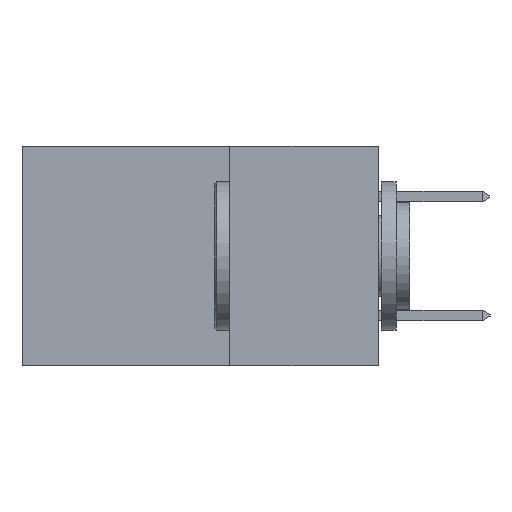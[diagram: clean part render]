
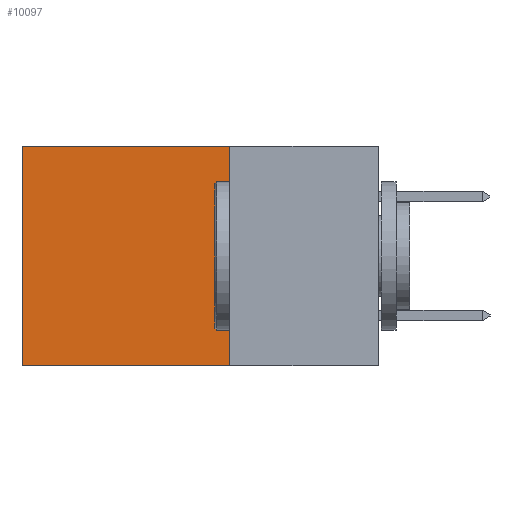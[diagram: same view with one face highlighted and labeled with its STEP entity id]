
A CAD part, left-side view. The second image highlights one B-rep face of the part: STEP entity #10097.
In plain terms, the highlighted planar face has unit normal (-1, 0, 0).
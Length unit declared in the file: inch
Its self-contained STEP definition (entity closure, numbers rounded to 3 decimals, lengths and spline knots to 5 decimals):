
#1505 = FACE_OUTER_BOUND ( 'NONE', #16225, .T. ) ;
#1739 = ORIENTED_EDGE ( 'NONE', *, *, #15482, .F. ) ;
#2769 = LINE ( 'NONE', #20878, #15574 ) ;
#2841 = EDGE_CURVE ( 'NONE', #17433, #18248, #5862, .T. ) ;
#3151 = LINE ( 'NONE', #16389, #19868 ) ;
#4175 = DIRECTION ( 'NONE',  ( 0., 1., 0. ) ) ;
#5307 = PLANE ( 'NONE',  #9100 ) ;
#5490 = VERTEX_POINT ( 'NONE', #20787 ) ;
#5681 = ORIENTED_EDGE ( 'NONE', *, *, #12714, .T. ) ;
#5862 = LINE ( 'NONE', #15817, #18675 ) ;
#6320 = CARTESIAN_POINT ( 'NONE',  ( 0.2615, 0.6, -0.37 ) ) ;
#7467 = CARTESIAN_POINT ( 'NONE',  ( 0.2615, 0.6, 0. ) ) ;
#8019 = DIRECTION ( 'NONE',  ( 0., 0., -1. ) ) ;
#8692 = DIRECTION ( 'NONE',  ( 0., 0., -1. ) ) ;
#8727 = LINE ( 'NONE', #6320, #17052 ) ;
#9100 = AXIS2_PLACEMENT_3D ( 'NONE', #16976, #18687, #8692 ) ;
#10097 = ADVANCED_FACE ( 'NONE', ( #1505 ), #5307, .F. ) ;
#11141 = EDGE_CURVE ( 'NONE', #5490, #21105, #2769, .T. ) ;
#12714 = EDGE_CURVE ( 'NONE', #18248, #21105, #8727, .T. ) ;
#13127 = DIRECTION ( 'NONE',  ( 0., 0., -1. ) ) ;
#15156 = ORIENTED_EDGE ( 'NONE', *, *, #2841, .T. ) ;
#15482 = EDGE_CURVE ( 'NONE', #17433, #5490, #3151, .T. ) ;
#15574 = VECTOR ( 'NONE', #4175, 39.37008 ) ;
#15602 = DIRECTION ( 'NONE',  ( 0., 1., 0. ) ) ;
#15817 = CARTESIAN_POINT ( 'NONE',  ( 0.2615, 0.25, 0. ) ) ;
#16225 = EDGE_LOOP ( 'NONE', ( #5681, #20166, #1739, #15156 ) ) ;
#16389 = CARTESIAN_POINT ( 'NONE',  ( 0.2615, 0.25, -0.37 ) ) ;
#16976 = CARTESIAN_POINT ( 'NONE',  ( 0.2615, 0.25, -0.37 ) ) ;
#17052 = VECTOR ( 'NONE', #8019, 39.37008 ) ;
#17433 = VERTEX_POINT ( 'NONE', #18635 ) ;
#17631 = CARTESIAN_POINT ( 'NONE',  ( 0.2615, 0.6, -0.37 ) ) ;
#18248 = VERTEX_POINT ( 'NONE', #7467 ) ;
#18635 = CARTESIAN_POINT ( 'NONE',  ( 0.2615, 0.25, 0. ) ) ;
#18675 = VECTOR ( 'NONE', #15602, 39.37008 ) ;
#18687 = DIRECTION ( 'NONE',  ( 1., 0., 0. ) ) ;
#19868 = VECTOR ( 'NONE', #13127, 39.37008 ) ;
#20166 = ORIENTED_EDGE ( 'NONE', *, *, #11141, .F. ) ;
#20787 = CARTESIAN_POINT ( 'NONE',  ( 0.2615, 0.25, -0.37 ) ) ;
#20878 = CARTESIAN_POINT ( 'NONE',  ( 0.2615, 0.25, -0.37 ) ) ;
#21105 = VERTEX_POINT ( 'NONE', #17631 ) ;
